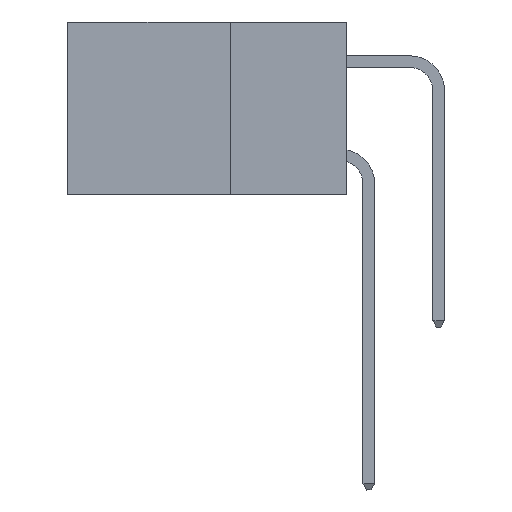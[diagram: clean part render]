
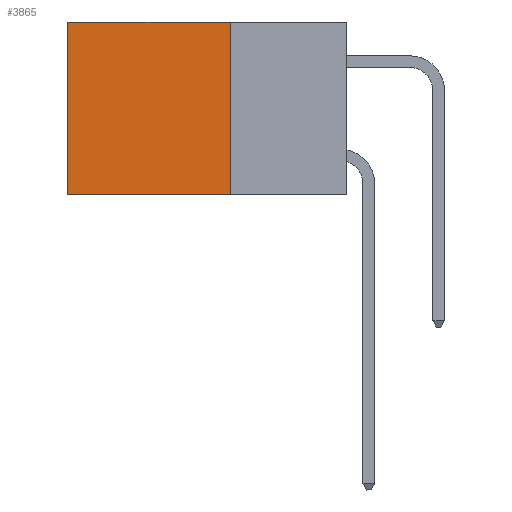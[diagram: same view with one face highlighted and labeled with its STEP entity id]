
A CAD part, left-side view. The second image highlights one B-rep face of the part: STEP entity #3865.
In plain terms, the highlighted planar face has unit normal (-1, 0, 0).
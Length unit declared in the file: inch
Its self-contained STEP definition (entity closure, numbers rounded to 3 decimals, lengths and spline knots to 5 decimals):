
#279 = DIRECTION ( 'NONE',  ( 1., 0., 0. ) ) ;
#1015 = VECTOR ( 'NONE', #9449, 39.37008 ) ;
#1663 = CARTESIAN_POINT ( 'NONE',  ( 0.2875, 0.25, 0. ) ) ;
#1772 = CARTESIAN_POINT ( 'NONE',  ( 0.2875, 0.25, -0.37 ) ) ;
#1952 = DIRECTION ( 'NONE',  ( 0., 0., -1. ) ) ;
#3083 = DIRECTION ( 'NONE',  ( 0., 0., -1. ) ) ;
#3865 = ADVANCED_FACE ( 'NONE', ( #7619 ), #7037, .F. ) ;
#4793 = DIRECTION ( 'NONE',  ( 0., 1., 0. ) ) ;
#4870 = AXIS2_PLACEMENT_3D ( 'NONE', #1663, #279, #3083 ) ;
#4990 = LINE ( 'NONE', #11514, #11820 ) ;
#5299 = EDGE_CURVE ( 'NONE', #16030, #16835, #4990, .T. ) ;
#5749 = CARTESIAN_POINT ( 'NONE',  ( 0.2875, 0.6, -0.37 ) ) ;
#5888 = EDGE_CURVE ( 'NONE', #15466, #13829, #9236, .T. ) ;
#6991 = EDGE_LOOP ( 'NONE', ( #11700, #13397, #14497, #7618 ) ) ;
#7037 = PLANE ( 'NONE',  #4870 ) ;
#7618 = ORIENTED_EDGE ( 'NONE', *, *, #8267, .T. ) ;
#7619 = FACE_OUTER_BOUND ( 'NONE', #6991, .T. ) ;
#8075 = CARTESIAN_POINT ( 'NONE',  ( 0.2875, 0.6, 0. ) ) ;
#8267 = EDGE_CURVE ( 'NONE', #16030, #15466, #8812, .T. ) ;
#8381 = VECTOR ( 'NONE', #4793, 39.37008 ) ;
#8391 = CARTESIAN_POINT ( 'NONE',  ( 0.2875, 0.25, 0. ) ) ;
#8812 = LINE ( 'NONE', #15575, #8381 ) ;
#9236 = LINE ( 'NONE', #8075, #13265 ) ;
#9449 = DIRECTION ( 'NONE',  ( 0., 1., 0. ) ) ;
#10638 = CARTESIAN_POINT ( 'NONE',  ( 0.2875, 0.25, -0.37 ) ) ;
#11514 = CARTESIAN_POINT ( 'NONE',  ( 0.2875, 0.25, 0. ) ) ;
#11648 = LINE ( 'NONE', #10638, #1015 ) ;
#11700 = ORIENTED_EDGE ( 'NONE', *, *, #5888, .T. ) ;
#11820 = VECTOR ( 'NONE', #1952, 39.37008 ) ;
#12396 = EDGE_CURVE ( 'NONE', #16835, #13829, #11648, .T. ) ;
#13265 = VECTOR ( 'NONE', #13988, 39.37008 ) ;
#13397 = ORIENTED_EDGE ( 'NONE', *, *, #12396, .F. ) ;
#13668 = CARTESIAN_POINT ( 'NONE',  ( 0.2875, 0.6, 0. ) ) ;
#13829 = VERTEX_POINT ( 'NONE', #5749 ) ;
#13988 = DIRECTION ( 'NONE',  ( 0., 0., -1. ) ) ;
#14497 = ORIENTED_EDGE ( 'NONE', *, *, #5299, .F. ) ;
#15466 = VERTEX_POINT ( 'NONE', #13668 ) ;
#15575 = CARTESIAN_POINT ( 'NONE',  ( 0.2875, 0.25, 0. ) ) ;
#16030 = VERTEX_POINT ( 'NONE', #8391 ) ;
#16835 = VERTEX_POINT ( 'NONE', #1772 ) ;
